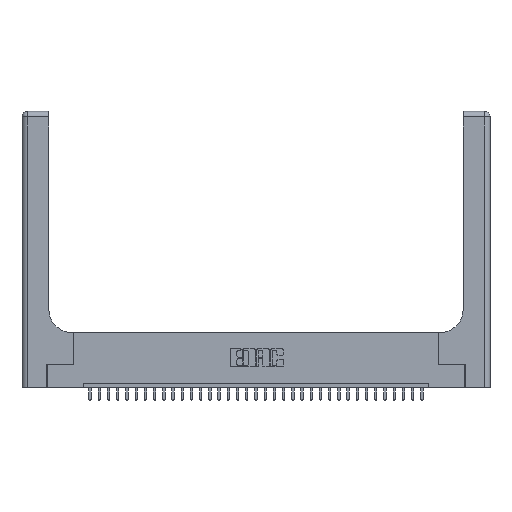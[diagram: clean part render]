
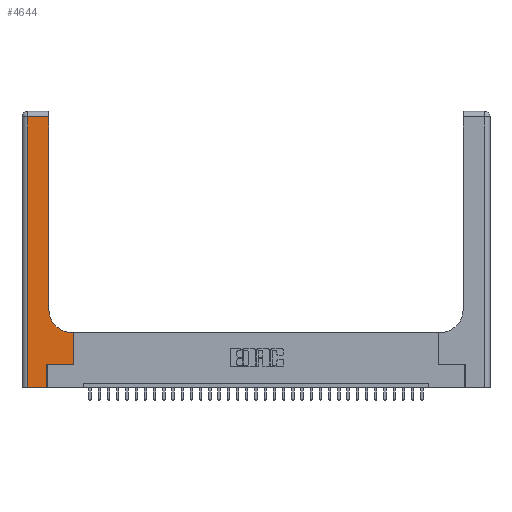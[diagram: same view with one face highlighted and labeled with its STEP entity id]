
A CAD part, top view. The second image highlights one B-rep face of the part: STEP entity #4644.
In plain terms, the highlighted planar face has unit normal (0, 0, 1).
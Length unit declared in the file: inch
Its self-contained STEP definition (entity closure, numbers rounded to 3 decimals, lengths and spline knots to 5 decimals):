
#77 = DIRECTION ( 'NONE',  ( 1., 0., 0. ) ) ;
#279 = CARTESIAN_POINT ( 'NONE',  ( 0.5585, 0.25, 0.37 ) ) ;
#622 = VERTEX_POINT ( 'NONE', #24687 ) ;
#1070 = LINE ( 'NONE', #28593, #18949 ) ;
#1250 = VECTOR ( 'NONE', #20261, 39.37008 ) ;
#1735 = DIRECTION ( 'NONE',  ( 1., 0., 0. ) ) ;
#3126 = CARTESIAN_POINT ( 'NONE',  ( 0.2915, 2.94, 0.37 ) ) ;
#3433 = EDGE_CURVE ( 'NONE', #30649, #12995, #4513, .T. ) ;
#3487 = EDGE_CURVE ( 'NONE', #31106, #30649, #10195, .T. ) ;
#3613 = VERTEX_POINT ( 'NONE', #3126 ) ;
#3702 = VECTOR ( 'NONE', #15794, 39.37008 ) ;
#3843 = AXIS2_PLACEMENT_3D ( 'NONE', #16162, #26129, #28871 ) ;
#3951 = VERTEX_POINT ( 'NONE', #18775 ) ;
#4105 = DIRECTION ( 'NONE',  ( 0., 1., 0. ) ) ;
#4513 = CIRCLE ( 'NONE', #9250, 0.25 ) ;
#4644 = ADVANCED_FACE ( 'NONE', ( #24734 ), #18542, .F. ) ;
#5419 = CARTESIAN_POINT ( 'NONE',  ( 0.06, 3., 0.37 ) ) ;
#5897 = DIRECTION ( 'NONE',  ( -1., 0., 0. ) ) ;
#6557 = LINE ( 'NONE', #32777, #31774 ) ;
#6778 = ORIENTED_EDGE ( 'NONE', *, *, #33140, .T. ) ;
#6951 = CARTESIAN_POINT ( 'NONE',  ( 0.06, 2.94, 0.37 ) ) ;
#6963 = ORIENTED_EDGE ( 'NONE', *, *, #3487, .T. ) ;
#7716 = CARTESIAN_POINT ( 'NONE',  ( 0.269, 0., 0.37 ) ) ;
#9248 = LINE ( 'NONE', #13640, #31252 ) ;
#9250 = AXIS2_PLACEMENT_3D ( 'NONE', #14910, #17159, #1735 ) ;
#9720 = CARTESIAN_POINT ( 'NONE',  ( 0.5415, 0.6, 0.37 ) ) ;
#10195 = LINE ( 'NONE', #30650, #1250 ) ;
#10570 = LINE ( 'NONE', #7716, #3702 ) ;
#12032 = EDGE_CURVE ( 'NONE', #3613, #20658, #9248, .T. ) ;
#12383 = CARTESIAN_POINT ( 'NONE',  ( 0., 0., 0.37 ) ) ;
#12995 = VERTEX_POINT ( 'NONE', #18767 ) ;
#13157 = DIRECTION ( 'NONE',  ( 0., -1., 0. ) ) ;
#13528 = ORIENTED_EDGE ( 'NONE', *, *, #26813, .T. ) ;
#13640 = CARTESIAN_POINT ( 'NONE',  ( 0., 2.94, 0.37 ) ) ;
#13684 = CARTESIAN_POINT ( 'NONE',  ( 0.06, 0., 0.37 ) ) ;
#14617 = ORIENTED_EDGE ( 'NONE', *, *, #20588, .T. ) ;
#14910 = CARTESIAN_POINT ( 'NONE',  ( 0.5415, 0.85, 0.37 ) ) ;
#15393 = EDGE_CURVE ( 'NONE', #12995, #3613, #6557, .T. ) ;
#15794 = DIRECTION ( 'NONE',  ( 0., 1., 0. ) ) ;
#16162 = CARTESIAN_POINT ( 'NONE',  ( 0., 3., 0.37 ) ) ;
#17159 = DIRECTION ( 'NONE',  ( 0., 0., -1. ) ) ;
#17501 = ORIENTED_EDGE ( 'NONE', *, *, #21551, .T. ) ;
#17649 = LINE ( 'NONE', #22000, #24976 ) ;
#18542 = PLANE ( 'NONE',  #3843 ) ;
#18767 = CARTESIAN_POINT ( 'NONE',  ( 0.2915, 0.85, 0.37 ) ) ;
#18775 = CARTESIAN_POINT ( 'NONE',  ( 0.269, 0., 0.37 ) ) ;
#18949 = VECTOR ( 'NONE', #77, 39.37008 ) ;
#19020 = LINE ( 'NONE', #12383, #28367 ) ;
#20261 = DIRECTION ( 'NONE',  ( -1., 0., 0. ) ) ;
#20588 = EDGE_CURVE ( 'NONE', #622, #28133, #1070, .T. ) ;
#20658 = VERTEX_POINT ( 'NONE', #6951 ) ;
#21551 = EDGE_CURVE ( 'NONE', #28133, #31106, #17649, .T. ) ;
#22000 = CARTESIAN_POINT ( 'NONE',  ( 0.5585, 0.25, 0.37 ) ) ;
#23370 = ORIENTED_EDGE ( 'NONE', *, *, #12032, .T. ) ;
#24687 = CARTESIAN_POINT ( 'NONE',  ( 0.269, 0.25, 0.37 ) ) ;
#24734 = FACE_OUTER_BOUND ( 'NONE', #30355, .T. ) ;
#24976 = VECTOR ( 'NONE', #27231, 39.37008 ) ;
#25595 = ORIENTED_EDGE ( 'NONE', *, *, #15393, .T. ) ;
#25750 = VERTEX_POINT ( 'NONE', #13684 ) ;
#26129 = DIRECTION ( 'NONE',  ( 0., 0., -1. ) ) ;
#26813 = EDGE_CURVE ( 'NONE', #20658, #25750, #28527, .T. ) ;
#27231 = DIRECTION ( 'NONE',  ( 0., 1., 0. ) ) ;
#27476 = CARTESIAN_POINT ( 'NONE',  ( 0.5585, 0.6, 0.37 ) ) ;
#28133 = VERTEX_POINT ( 'NONE', #279 ) ;
#28365 = DIRECTION ( 'NONE',  ( 1., 0., 0. ) ) ;
#28367 = VECTOR ( 'NONE', #28365, 39.37008 ) ;
#28527 = LINE ( 'NONE', #5419, #33494 ) ;
#28593 = CARTESIAN_POINT ( 'NONE',  ( 0.269, 0.25, 0.37 ) ) ;
#28871 = DIRECTION ( 'NONE',  ( -1., 0., 0. ) ) ;
#30355 = EDGE_LOOP ( 'NONE', ( #25595, #23370, #13528, #6778, #32563, #14617, #17501, #6963, #32987 ) ) ;
#30649 = VERTEX_POINT ( 'NONE', #9720 ) ;
#30650 = CARTESIAN_POINT ( 'NONE',  ( 0.2915, 0.6, 0.37 ) ) ;
#30843 = EDGE_CURVE ( 'NONE', #3951, #622, #10570, .T. ) ;
#31106 = VERTEX_POINT ( 'NONE', #27476 ) ;
#31252 = VECTOR ( 'NONE', #5897, 39.37008 ) ;
#31774 = VECTOR ( 'NONE', #4105, 39.37008 ) ;
#32563 = ORIENTED_EDGE ( 'NONE', *, *, #30843, .T. ) ;
#32777 = CARTESIAN_POINT ( 'NONE',  ( 0.2915, 3., 0.37 ) ) ;
#32987 = ORIENTED_EDGE ( 'NONE', *, *, #3433, .T. ) ;
#33140 = EDGE_CURVE ( 'NONE', #25750, #3951, #19020, .T. ) ;
#33494 = VECTOR ( 'NONE', #13157, 39.37008 ) ;
